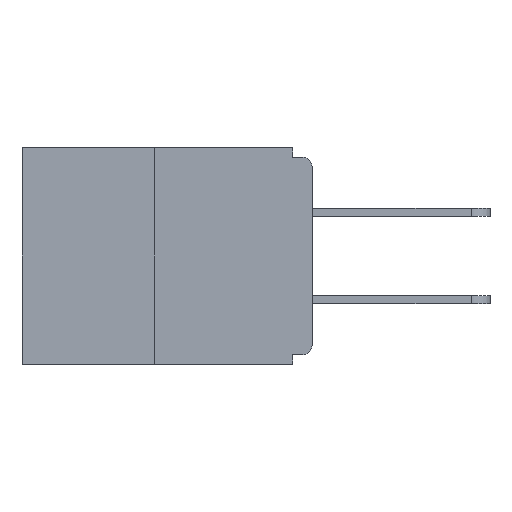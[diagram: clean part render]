
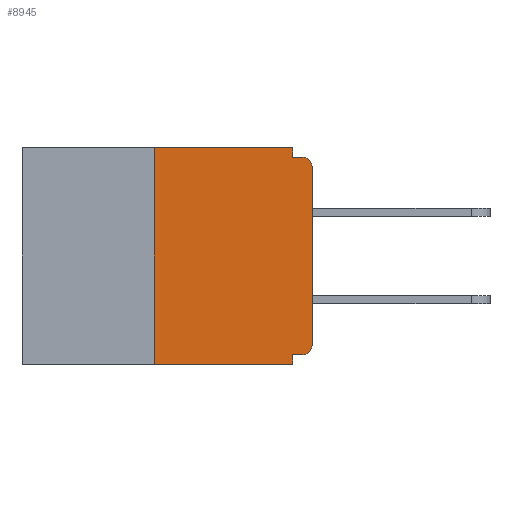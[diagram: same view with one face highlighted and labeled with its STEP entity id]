
A CAD part, left-side view. The second image highlights one B-rep face of the part: STEP entity #8945.
In plain terms, the highlighted planar face has unit normal (-1, 0, 0).
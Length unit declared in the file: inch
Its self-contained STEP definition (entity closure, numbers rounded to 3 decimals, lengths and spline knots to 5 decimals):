
#80 = EDGE_CURVE ( 'NONE', #7305, #7093, #8789, .T. ) ;
#134 = CARTESIAN_POINT ( 'NONE',  ( 0., 0.015, -0.03 ) ) ;
#435 = AXIS2_PLACEMENT_3D ( 'NONE', #11263, #11143, #11319 ) ;
#779 = CARTESIAN_POINT ( 'NONE',  ( 0., 0., 0. ) ) ;
#837 = CARTESIAN_POINT ( 'NONE',  ( 0., 0.46, 0. ) ) ;
#1573 = CARTESIAN_POINT ( 'NONE',  ( 0., 0.015, -0.328 ) ) ;
#1598 = EDGE_CURVE ( 'NONE', #6940, #7305, #1701, .T. ) ;
#1701 = LINE ( 'NONE', #779, #15998 ) ;
#1791 = CARTESIAN_POINT ( 'NONE',  ( 0., 0.015, -0.015 ) ) ;
#1920 = LINE ( 'NONE', #837, #4867 ) ;
#2318 = DIRECTION ( 'NONE',  ( 0., -1., 0. ) ) ;
#2411 = CARTESIAN_POINT ( 'NONE',  ( 0., 0.031, 0. ) ) ;
#2505 = CARTESIAN_POINT ( 'NONE',  ( 0., 0., -0.015 ) ) ;
#2519 = EDGE_CURVE ( 'NONE', #3320, #6940, #5999, .T. ) ;
#2588 = ORIENTED_EDGE ( 'NONE', *, *, #2519, .T. ) ;
#2596 = CARTESIAN_POINT ( 'NONE',  ( 0., 0.25, 0. ) ) ;
#2629 = EDGE_CURVE ( 'NONE', #8843, #9369, #18543, .T. ) ;
#3077 = ORIENTED_EDGE ( 'NONE', *, *, #12711, .F. ) ;
#3109 = CARTESIAN_POINT ( 'NONE',  ( 0., 0., -0.328 ) ) ;
#3320 = VERTEX_POINT ( 'NONE', #1573 ) ;
#3444 = VECTOR ( 'NONE', #8811, 39.37008 ) ;
#3714 = DIRECTION ( 'NONE',  ( 0., 0., 1. ) ) ;
#3731 = VECTOR ( 'NONE', #18493, 39.37008 ) ;
#3917 = CARTESIAN_POINT ( 'NONE',  ( 0., 0.25, 0. ) ) ;
#4016 = CARTESIAN_POINT ( 'NONE',  ( 0., 0.25, -0.343 ) ) ;
#4075 = DIRECTION ( 'NONE',  ( -1., 0., 0. ) ) ;
#4357 = EDGE_CURVE ( 'NONE', #17671, #8843, #1920, .T. ) ;
#4461 = EDGE_CURVE ( 'NONE', #9369, #7093, #14579, .T. ) ;
#4780 = ORIENTED_EDGE ( 'NONE', *, *, #2629, .F. ) ;
#4845 = DIRECTION ( 'NONE',  ( 0., 0., -1. ) ) ;
#4867 = VECTOR ( 'NONE', #13878, 39.37008 ) ;
#5056 = CARTESIAN_POINT ( 'NONE',  ( 0., 0.031, -0.343 ) ) ;
#5206 = ORIENTED_EDGE ( 'NONE', *, *, #4461, .F. ) ;
#5580 = CARTESIAN_POINT ( 'NONE',  ( 0., 0.031, -0.328 ) ) ;
#5725 = EDGE_CURVE ( 'NONE', #3320, #6155, #15449, .T. ) ;
#5993 = ORIENTED_EDGE ( 'NONE', *, *, #80, .T. ) ;
#5999 = CIRCLE ( 'NONE', #17521, 0.015 ) ;
#6155 = VERTEX_POINT ( 'NONE', #5580 ) ;
#6503 = DIRECTION ( 'NONE',  ( 0., 0., -1. ) ) ;
#6940 = VERTEX_POINT ( 'NONE', #9894 ) ;
#7093 = VERTEX_POINT ( 'NONE', #1791 ) ;
#7305 = VERTEX_POINT ( 'NONE', #10823 ) ;
#7319 = DIRECTION ( 'NONE',  ( -1., 0., 0. ) ) ;
#7440 = LINE ( 'NONE', #14131, #10360 ) ;
#8630 = CARTESIAN_POINT ( 'NONE',  ( 0., 0.031, 0. ) ) ;
#8789 = CIRCLE ( 'NONE', #13811, 0.015 ) ;
#8811 = DIRECTION ( 'NONE',  ( 0., 1., 0. ) ) ;
#8843 = VERTEX_POINT ( 'NONE', #2411 ) ;
#8945 = ADVANCED_FACE ( 'NONE', ( #15186 ), #12841, .F. ) ;
#9369 = VERTEX_POINT ( 'NONE', #15492 ) ;
#9894 = CARTESIAN_POINT ( 'NONE',  ( 0., 0., -0.313 ) ) ;
#10360 = VECTOR ( 'NONE', #2318, 39.37008 ) ;
#10462 = EDGE_CURVE ( 'NONE', #6155, #12102, #16995, .T. ) ;
#10735 = VECTOR ( 'NONE', #14201, 39.37008 ) ;
#10804 = VECTOR ( 'NONE', #14377, 39.37008 ) ;
#10823 = CARTESIAN_POINT ( 'NONE',  ( 0., 0., -0.03 ) ) ;
#10976 = LINE ( 'NONE', #3917, #3731 ) ;
#11143 = DIRECTION ( 'NONE',  ( 1., 0., 0. ) ) ;
#11244 = ORIENTED_EDGE ( 'NONE', *, *, #4357, .F. ) ;
#11263 = CARTESIAN_POINT ( 'NONE',  ( 0., 0.46, 0. ) ) ;
#11319 = DIRECTION ( 'NONE',  ( 0., 0., -1. ) ) ;
#11686 = VERTEX_POINT ( 'NONE', #4016 ) ;
#12102 = VERTEX_POINT ( 'NONE', #12669 ) ;
#12669 = CARTESIAN_POINT ( 'NONE',  ( 0., 0.031, -0.343 ) ) ;
#12711 = EDGE_CURVE ( 'NONE', #11686, #17671, #10976, .T. ) ;
#12841 = PLANE ( 'NONE',  #435 ) ;
#13811 = AXIS2_PLACEMENT_3D ( 'NONE', #134, #7319, #4845 ) ;
#13878 = DIRECTION ( 'NONE',  ( 0., -1., 0. ) ) ;
#14013 = ORIENTED_EDGE ( 'NONE', *, *, #10462, .F. ) ;
#14063 = DIRECTION ( 'NONE',  ( 0., 0., -1. ) ) ;
#14127 = CARTESIAN_POINT ( 'NONE',  ( 0., 0.015, -0.313 ) ) ;
#14131 = CARTESIAN_POINT ( 'NONE',  ( 0., 0.46, -0.343 ) ) ;
#14201 = DIRECTION ( 'NONE',  ( 0., -1., 0. ) ) ;
#14377 = DIRECTION ( 'NONE',  ( 0., 0., -1. ) ) ;
#14579 = LINE ( 'NONE', #2505, #10735 ) ;
#14691 = ORIENTED_EDGE ( 'NONE', *, *, #18734, .T. ) ;
#15186 = FACE_OUTER_BOUND ( 'NONE', #17613, .T. ) ;
#15449 = LINE ( 'NONE', #3109, #3444 ) ;
#15492 = CARTESIAN_POINT ( 'NONE',  ( 0., 0.031, -0.015 ) ) ;
#15814 = ORIENTED_EDGE ( 'NONE', *, *, #5725, .F. ) ;
#15998 = VECTOR ( 'NONE', #3714, 39.37008 ) ;
#16302 = VECTOR ( 'NONE', #6503, 39.37008 ) ;
#16995 = LINE ( 'NONE', #5056, #16302 ) ;
#17260 = ORIENTED_EDGE ( 'NONE', *, *, #1598, .T. ) ;
#17521 = AXIS2_PLACEMENT_3D ( 'NONE', #14127, #4075, #14063 ) ;
#17613 = EDGE_LOOP ( 'NONE', ( #11244, #3077, #14691, #14013, #15814, #2588, #17260, #5993, #5206, #4780 ) ) ;
#17671 = VERTEX_POINT ( 'NONE', #2596 ) ;
#18493 = DIRECTION ( 'NONE',  ( 0., 0., 1. ) ) ;
#18543 = LINE ( 'NONE', #8630, #10804 ) ;
#18734 = EDGE_CURVE ( 'NONE', #11686, #12102, #7440, .T. ) ;
